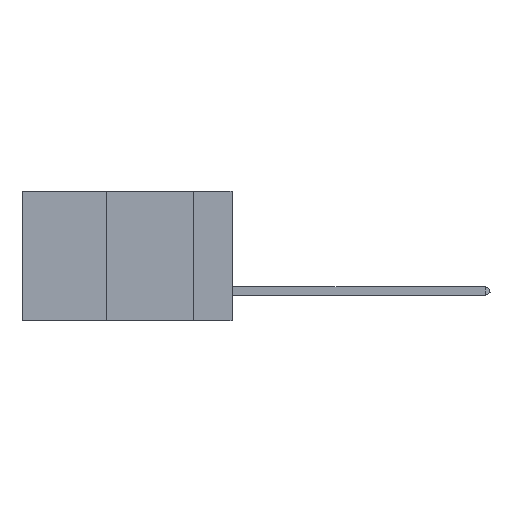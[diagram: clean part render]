
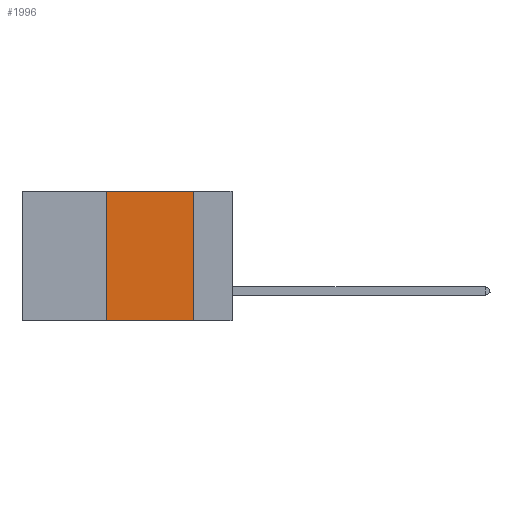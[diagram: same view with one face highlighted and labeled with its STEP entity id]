
A CAD part, left-side view. The second image highlights one B-rep face of the part: STEP entity #1996.
In plain terms, the highlighted planar face has unit normal (-1, 0, 0).
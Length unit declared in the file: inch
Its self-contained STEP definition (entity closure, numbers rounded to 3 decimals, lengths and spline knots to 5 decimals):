
#54 = CARTESIAN_POINT ( 'NONE',  ( 0., 0.11, 0. ) ) ;
#84 = CARTESIAN_POINT ( 'NONE',  ( 0., 0.6, -0.37 ) ) ;
#1226 = EDGE_CURVE ( 'NONE', #5074, #6269, #9746, .T. ) ;
#1738 = ORIENTED_EDGE ( 'NONE', *, *, #2865, .F. ) ;
#1996 = ADVANCED_FACE ( 'NONE', ( #5219 ), #12031, .F. ) ;
#2302 = DIRECTION ( 'NONE',  ( 1., 0., 0. ) ) ;
#2795 = CARTESIAN_POINT ( 'NONE',  ( 0., 0.36, -0.37 ) ) ;
#2865 = EDGE_CURVE ( 'NONE', #13730, #9407, #6064, .T. ) ;
#5074 = VERTEX_POINT ( 'NONE', #2795 ) ;
#5219 = FACE_OUTER_BOUND ( 'NONE', #11576, .T. ) ;
#5369 = AXIS2_PLACEMENT_3D ( 'NONE', #13189, #2302, #16050 ) ;
#5823 = ORIENTED_EDGE ( 'NONE', *, *, #1226, .F. ) ;
#6064 = LINE ( 'NONE', #54, #17536 ) ;
#6269 = VERTEX_POINT ( 'NONE', #12636 ) ;
#6662 = EDGE_CURVE ( 'NONE', #6269, #13730, #7207, .T. ) ;
#6705 = DIRECTION ( 'NONE',  ( 0., -1., 0. ) ) ;
#6843 = EDGE_CURVE ( 'NONE', #5074, #9407, #16727, .T. ) ;
#7207 = LINE ( 'NONE', #10754, #16517 ) ;
#8898 = ORIENTED_EDGE ( 'NONE', *, *, #6662, .F. ) ;
#8915 = VECTOR ( 'NONE', #11058, 39.37008 ) ;
#9407 = VERTEX_POINT ( 'NONE', #11852 ) ;
#9746 = LINE ( 'NONE', #15174, #17354 ) ;
#9753 = DIRECTION ( 'NONE',  ( 0., 0., -1. ) ) ;
#10754 = CARTESIAN_POINT ( 'NONE',  ( 0., 0.6, 0. ) ) ;
#11058 = DIRECTION ( 'NONE',  ( 0., -1., 0. ) ) ;
#11576 = EDGE_LOOP ( 'NONE', ( #1738, #8898, #5823, #12185 ) ) ;
#11852 = CARTESIAN_POINT ( 'NONE',  ( 0., 0.11, -0.37 ) ) ;
#12031 = PLANE ( 'NONE',  #5369 ) ;
#12185 = ORIENTED_EDGE ( 'NONE', *, *, #6843, .T. ) ;
#12359 = DIRECTION ( 'NONE',  ( 0., 0., 1. ) ) ;
#12636 = CARTESIAN_POINT ( 'NONE',  ( 0., 0.36, 0. ) ) ;
#13189 = CARTESIAN_POINT ( 'NONE',  ( 0., 0.6, 0. ) ) ;
#13730 = VERTEX_POINT ( 'NONE', #17745 ) ;
#15174 = CARTESIAN_POINT ( 'NONE',  ( 0., 0.36, 0. ) ) ;
#16050 = DIRECTION ( 'NONE',  ( 0., 0., -1. ) ) ;
#16517 = VECTOR ( 'NONE', #6705, 39.37008 ) ;
#16727 = LINE ( 'NONE', #84, #8915 ) ;
#17354 = VECTOR ( 'NONE', #12359, 39.37008 ) ;
#17536 = VECTOR ( 'NONE', #9753, 39.37008 ) ;
#17745 = CARTESIAN_POINT ( 'NONE',  ( 0., 0.11, 0. ) ) ;
